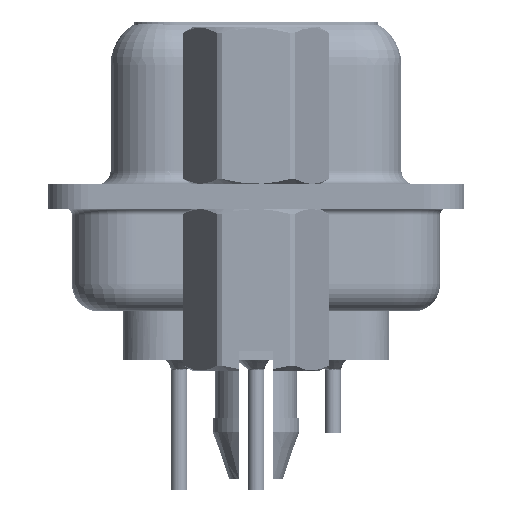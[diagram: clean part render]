
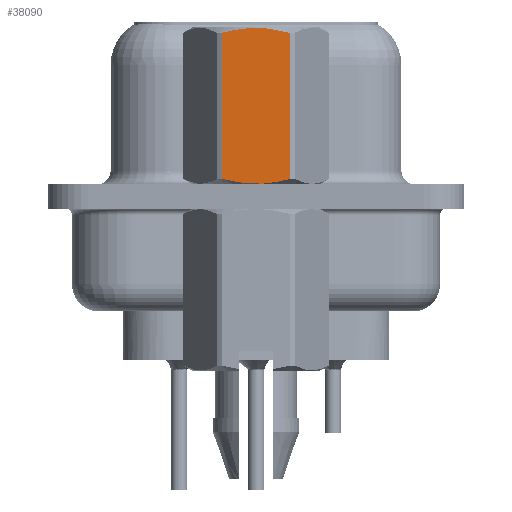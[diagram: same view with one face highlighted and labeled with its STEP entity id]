
A CAD part, left-side view. The second image highlights one B-rep face of the part: STEP entity #38090.
In plain terms, the highlighted planar face has unit normal (-1, 0, 0).
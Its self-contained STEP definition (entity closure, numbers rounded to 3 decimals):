
#5764 = CARTESIAN_POINT ( 'NONE',  ( -2.381, -0.432, 0.485 ) ) ;
#5798 = CARTESIAN_POINT ( 'NONE',  ( -2.381, 1.273, 3.792 ) ) ;
#8926 = CARTESIAN_POINT ( 'NONE',  ( -2.381, -1.273, 0.652 ) ) ;
#9043 = DIRECTION ( 'NONE',  ( 0., 0., 1. ) ) ;
#9160 = CARTESIAN_POINT ( 'NONE',  ( -2.381, 0.215, 0.468 ) ) ;
#11252 = ORIENTED_EDGE ( 'NONE', *, *, #20187, .T. ) ;
#12155 = CARTESIAN_POINT ( 'NONE',  ( -2.381, 1.273, 0.652 ) ) ;
#12237 = CARTESIAN_POINT ( 'NONE',  ( -2.381, -1.273, 3.792 ) ) ;
#13074 = CARTESIAN_POINT ( 'NONE',  ( -2.381, 0.428, 0.485 ) ) ;
#14351 = CARTESIAN_POINT ( 'NONE',  ( -2.381, -0.432, 6.215 ) ) ;
#14585 = CARTESIAN_POINT ( 'NONE',  ( -2.381, 0.215, 6.232 ) ) ;
#17985 = CARTESIAN_POINT ( 'NONE',  ( -2.381, -1.273, 6.048 ) ) ;
#20187 = EDGE_CURVE ( 'NONE', #30074, #28537, #27242, .T. ) ;
#21048 = FACE_OUTER_BOUND ( 'NONE', #48250, .T. ) ;
#23068 = CARTESIAN_POINT ( 'NONE',  ( -2.381, -1.273, 0.652 ) ) ;
#23486 = ORIENTED_EDGE ( 'NONE', *, *, #26032, .T. ) ;
#23586 = CARTESIAN_POINT ( 'NONE',  ( -2.381, -0.215, 0.468 ) ) ;
#24551 = CARTESIAN_POINT ( 'NONE',  ( -2.381, 1.065, 0.596 ) ) ;
#24618 = CARTESIAN_POINT ( 'NONE',  ( -2.381, 1.065, 6.104 ) ) ;
#24855 = CARTESIAN_POINT ( 'NONE',  ( -2.381, 0.853, 6.151 ) ) ;
#24971 = CARTESIAN_POINT ( 'NONE',  ( -2.381, 1.375, -3.75 ) ) ;
#26032 = EDGE_CURVE ( 'NONE', #34680, #43635, #26877, .T. ) ;
#26877 = B_SPLINE_CURVE_WITH_KNOTS ( 'NONE', 3,
 ( #17985, #32871, #47830, #14351, #48065, #14585, #44404, #24855, #24618, #39500 ),
 .UNSPECIFIED., .F., .F.,
 ( 4, 2, 2, 2, 4 ),
 ( 0.001, 0.002, 0.002, 0.003, 0.004 ),
 .UNSPECIFIED. ) ;
#27242 = B_SPLINE_CURVE_WITH_KNOTS ( 'NONE', 3,
 ( #27473, #24551, #42888, #13074, #9160, #23586, #5764, #31603, #42414, #8926 ),
 .UNSPECIFIED., .F., .F.,
 ( 4, 2, 2, 2, 4 ),
 ( 0.003, 0.003, 0.004, 0.004, 0.005 ),
 .UNSPECIFIED. ) ;
#27473 = CARTESIAN_POINT ( 'NONE',  ( -2.381, 1.273, 0.652 ) ) ;
#28537 = VERTEX_POINT ( 'NONE', #23068 ) ;
#28615 = CARTESIAN_POINT ( 'NONE',  ( -2.381, -1.273, 6.048 ) ) ;
#30045 = DIRECTION ( 'NONE',  ( -1., 0., 0. ) ) ;
#30074 = VERTEX_POINT ( 'NONE', #12155 ) ;
#31603 = CARTESIAN_POINT ( 'NONE',  ( -2.381, -0.858, 0.55 ) ) ;
#32660 = EDGE_CURVE ( 'NONE', #28537, #34680, #42523, .T. ) ;
#32871 = CARTESIAN_POINT ( 'NONE',  ( -2.381, -1.066, 6.104 ) ) ;
#34680 = VERTEX_POINT ( 'NONE', #28615 ) ;
#35007 = CARTESIAN_POINT ( 'NONE',  ( -2.381, 1.273, 6.048 ) ) ;
#35930 = PLANE ( 'NONE',  #45025 ) ;
#38090 = ADVANCED_FACE ( 'NONE', ( #21048 ), #35930, .T. ) ;
#38851 = VECTOR ( 'NONE', #39237, 1000. ) ;
#38976 = LINE ( 'NONE', #5798, #38851 ) ;
#39237 = DIRECTION ( 'NONE',  ( 0., 0., -1. ) ) ;
#39500 = CARTESIAN_POINT ( 'NONE',  ( -2.381, 1.273, 6.048 ) ) ;
#40846 = DIRECTION ( 'NONE',  ( 0., -1., 0. ) ) ;
#41354 = EDGE_CURVE ( 'NONE', #43635, #30074, #38976, .T. ) ;
#41410 = ORIENTED_EDGE ( 'NONE', *, *, #41354, .T. ) ;
#42414 = CARTESIAN_POINT ( 'NONE',  ( -2.381, -1.066, 0.596 ) ) ;
#42523 = LINE ( 'NONE', #12237, #47840 ) ;
#42888 = CARTESIAN_POINT ( 'NONE',  ( -2.381, 0.853, 0.549 ) ) ;
#43635 = VERTEX_POINT ( 'NONE', #35007 ) ;
#44404 = CARTESIAN_POINT ( 'NONE',  ( -2.381, 0.428, 6.215 ) ) ;
#44758 = ORIENTED_EDGE ( 'NONE', *, *, #32660, .T. ) ;
#45025 = AXIS2_PLACEMENT_3D ( 'NONE', #24971, #30045, #40846 ) ;
#47830 = CARTESIAN_POINT ( 'NONE',  ( -2.381, -0.858, 6.15 ) ) ;
#47840 = VECTOR ( 'NONE', #9043, 1000. ) ;
#48065 = CARTESIAN_POINT ( 'NONE',  ( -2.381, -0.215, 6.232 ) ) ;
#48250 = EDGE_LOOP ( 'NONE', ( #11252, #44758, #23486, #41410 ) ) ;
